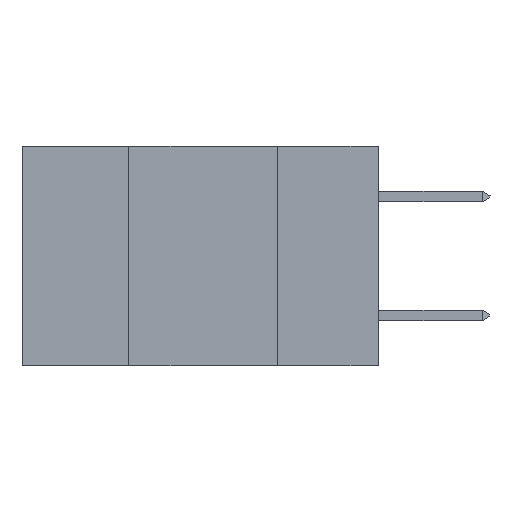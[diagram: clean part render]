
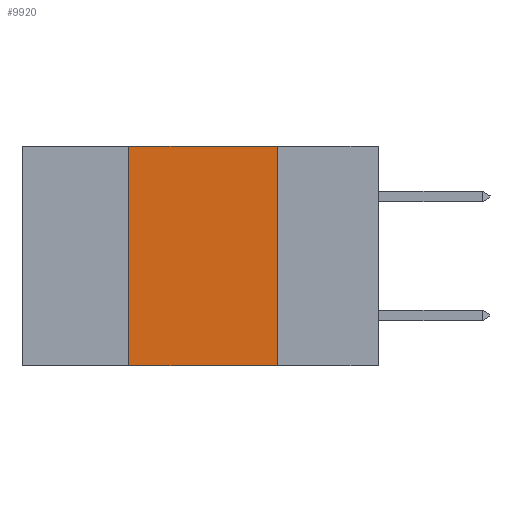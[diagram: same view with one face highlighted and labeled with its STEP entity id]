
A CAD part, left-side view. The second image highlights one B-rep face of the part: STEP entity #9920.
In plain terms, the highlighted planar face has unit normal (-1, 0, 0).
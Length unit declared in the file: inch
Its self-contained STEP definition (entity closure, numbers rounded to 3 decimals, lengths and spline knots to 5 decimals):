
#390 = VERTEX_POINT ( 'NONE', #4663 ) ;
#1204 = DIRECTION ( 'NONE',  ( 0., 0., -1. ) ) ;
#1298 = VERTEX_POINT ( 'NONE', #8440 ) ;
#1598 = DIRECTION ( 'NONE',  ( 0., 0., -1. ) ) ;
#1844 = VECTOR ( 'NONE', #1204, 39.37008 ) ;
#2060 = ORIENTED_EDGE ( 'NONE', *, *, #6917, .T. ) ;
#2271 = CARTESIAN_POINT ( 'NONE',  ( 0., 0.42, -0.37 ) ) ;
#2440 = VERTEX_POINT ( 'NONE', #7128 ) ;
#2567 = AXIS2_PLACEMENT_3D ( 'NONE', #4439, #5276, #1598 ) ;
#2873 = CARTESIAN_POINT ( 'NONE',  ( 0., 0.17, -0.37 ) ) ;
#3301 = ORIENTED_EDGE ( 'NONE', *, *, #8089, .F. ) ;
#3372 = PLANE ( 'NONE',  #2567 ) ;
#3487 = DIRECTION ( 'NONE',  ( 0., 0., 1. ) ) ;
#4253 = CARTESIAN_POINT ( 'NONE',  ( 0., 0.6, -0.37 ) ) ;
#4399 = ORIENTED_EDGE ( 'NONE', *, *, #8166, .F. ) ;
#4439 = CARTESIAN_POINT ( 'NONE',  ( 0., 0.6, 0. ) ) ;
#4451 = LINE ( 'NONE', #9067, #8485 ) ;
#4663 = CARTESIAN_POINT ( 'NONE',  ( 0., 0.17, -0.37 ) ) ;
#4925 = VECTOR ( 'NONE', #10312, 39.37008 ) ;
#4982 = EDGE_CURVE ( 'NONE', #2440, #390, #9085, .T. ) ;
#5276 = DIRECTION ( 'NONE',  ( 1., 0., 0. ) ) ;
#6390 = DIRECTION ( 'NONE',  ( 0., -1., 0. ) ) ;
#6438 = VECTOR ( 'NONE', #3487, 39.37008 ) ;
#6917 = EDGE_CURVE ( 'NONE', #6976, #390, #8772, .T. ) ;
#6976 = VERTEX_POINT ( 'NONE', #2271 ) ;
#7033 = FACE_OUTER_BOUND ( 'NONE', #7923, .T. ) ;
#7128 = CARTESIAN_POINT ( 'NONE',  ( 0., 0.17, 0. ) ) ;
#7923 = EDGE_LOOP ( 'NONE', ( #8193, #3301, #4399, #2060 ) ) ;
#8089 = EDGE_CURVE ( 'NONE', #1298, #2440, #4451, .T. ) ;
#8166 = EDGE_CURVE ( 'NONE', #6976, #1298, #8899, .T. ) ;
#8193 = ORIENTED_EDGE ( 'NONE', *, *, #4982, .F. ) ;
#8440 = CARTESIAN_POINT ( 'NONE',  ( 0., 0.42, 0. ) ) ;
#8485 = VECTOR ( 'NONE', #6390, 39.37008 ) ;
#8772 = LINE ( 'NONE', #4253, #4925 ) ;
#8899 = LINE ( 'NONE', #9872, #6438 ) ;
#9067 = CARTESIAN_POINT ( 'NONE',  ( 0., 0.6, 0. ) ) ;
#9085 = LINE ( 'NONE', #2873, #1844 ) ;
#9872 = CARTESIAN_POINT ( 'NONE',  ( 0., 0.42, -0.37 ) ) ;
#9920 = ADVANCED_FACE ( 'NONE', ( #7033 ), #3372, .F. ) ;
#10312 = DIRECTION ( 'NONE',  ( 0., -1., 0. ) ) ;
